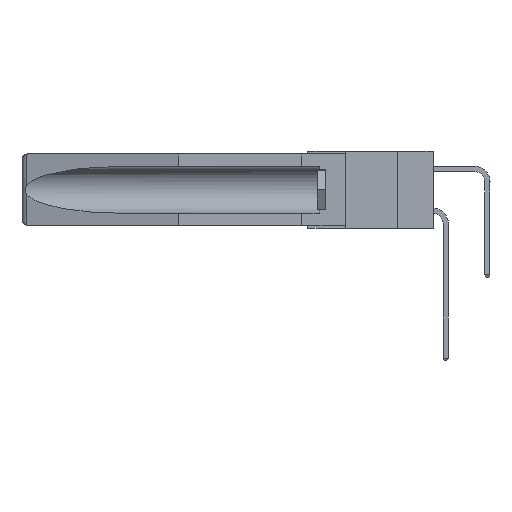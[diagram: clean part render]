
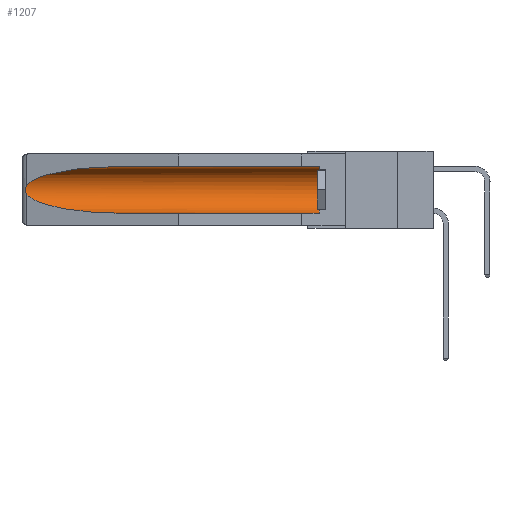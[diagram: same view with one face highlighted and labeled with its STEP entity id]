
A CAD part, left-side view. The second image highlights one B-rep face of the part: STEP entity #1207.
In plain terms, the highlighted cylindrical face has radius 2.857 mm (diameter 5.715 mm), a partial arc.
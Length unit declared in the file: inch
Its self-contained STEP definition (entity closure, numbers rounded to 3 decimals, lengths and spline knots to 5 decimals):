
#34 = CARTESIAN_POINT ( 'NONE',  ( 0.26655, 1.53094, -0.18657 ) ) ;
#533 = CARTESIAN_POINT ( 'NONE',  ( 0.155, 0.126, -0.059 ) ) ;
#949 = VERTEX_POINT ( 'NONE', #533 ) ;
#1207 = ADVANCED_FACE ( 'NONE', ( #13587 ), #18094, .F. ) ;
#1310 = CARTESIAN_POINT ( 'NONE',  ( 0.155, 0.126, -0.284 ) ) ;
#1577 = CARTESIAN_POINT ( 'NONE',  ( 0.26597, 1.5296, -0.19026 ) ) ;
#2385 = CARTESIAN_POINT ( 'NONE',  ( 0.155, 1.07973, -0.059 ) ) ;
#2899 = CARTESIAN_POINT ( 'NONE',  ( 0.2675, 1.53308, -0.16763 ) ) ;
#3165 = CARTESIAN_POINT ( 'NONE',  ( 0.26597, 1.52961, -0.15275 ) ) ;
#3187 =( BOUNDED_CURVE ( )  B_SPLINE_CURVE ( 3, ( #5237, #18400, #6705, #9602 ),
 .UNSPECIFIED., .F., .F. ) 
 B_SPLINE_CURVE_WITH_KNOTS ( ( 4, 4 ),
 ( 0.1948, 1.5708 ),
 .UNSPECIFIED. ) 
 CURVE ( )  GEOMETRIC_REPRESENTATION_ITEM ( )  RATIONAL_B_SPLINE_CURVE ( ( 1., 0.848, 0.848, 1. ) ) 
 REPRESENTATION_ITEM ( '' )  );
#3594 = ORIENTED_EDGE ( 'NONE', *, *, #14632, .T. ) ;
#4038 = CARTESIAN_POINT ( 'NONE',  ( 0.155, 1.07973, -0.059 ) ) ;
#4107 = DIRECTION ( 'NONE',  ( 0., 0., 1. ) ) ;
#4496 = CARTESIAN_POINT ( 'NONE',  ( 0.26537, 1.52718, -0.19328 ) ) ;
#5037 = CIRCLE ( 'NONE', #17253, 0.1125 ) ;
#5213 = ORIENTED_EDGE ( 'NONE', *, *, #16101, .T. ) ;
#5237 = CARTESIAN_POINT ( 'NONE',  ( 0.26537, 1.52718, -0.19328 ) ) ;
#5272 = CARTESIAN_POINT ( 'NONE',  ( 0.21114, 1.30732, -0.059 ) ) ;
#6705 = CARTESIAN_POINT ( 'NONE',  ( 0.21114, 1.30732, -0.284 ) ) ;
#7169 = VERTEX_POINT ( 'NONE', #14437 ) ;
#7429 = CARTESIAN_POINT ( 'NONE',  ( 0.155, -0.30754, -0.1715 ) ) ;
#7933 = CARTESIAN_POINT ( 'NONE',  ( 0.155, -0.30754, -0.284 ) ) ;
#8153 = CARTESIAN_POINT ( 'NONE',  ( 0.26537, 1.52718, -0.14972 ) ) ;
#8273 = CARTESIAN_POINT ( 'NONE',  ( 0.25451, 1.48313, -0.09465 ) ) ;
#8416 = EDGE_CURVE ( 'NONE', #9540, #18323, #3187, .T. ) ;
#8441 = ORIENTED_EDGE ( 'NONE', *, *, #12643, .T. ) ;
#8804 = DIRECTION ( 'NONE',  ( 0., 0., 1. ) ) ;
#9417 = VECTOR ( 'NONE', #18021, 39.37008 ) ;
#9540 = VERTEX_POINT ( 'NONE', #13170 ) ;
#9602 = CARTESIAN_POINT ( 'NONE',  ( 0.155, 1.07973, -0.284 ) ) ;
#9893 = DIRECTION ( 'NONE',  ( 0., -1., 0. ) ) ;
#10292 = CARTESIAN_POINT ( 'NONE',  ( 0.2673, 1.53269, -0.17917 ) ) ;
#10421 = CARTESIAN_POINT ( 'NONE',  ( 0.2675, 1.53308, -0.17534 ) ) ;
#11220 = ORIENTED_EDGE ( 'NONE', *, *, #12162, .F. ) ;
#11385 = B_SPLINE_CURVE_WITH_KNOTS ( 'NONE', 3,
 ( #17722, #3165, #17658, #13363, #2899, #10421, #10292, #34, #1577, #4496 ),
 .UNSPECIFIED., .F., .F.,
 ( 4, 2, 2, 2, 4 ),
 ( 0., 0.00029, 0.00058, 0.00087, 0.00117 ),
 .UNSPECIFIED. ) ;
#11499 = CARTESIAN_POINT ( 'NONE',  ( 0.155, 0.126, -0.1715 ) ) ;
#11554 = EDGE_CURVE ( 'NONE', #949, #14743, #14263, .T. ) ;
#12162 = EDGE_CURVE ( 'NONE', #16136, #18323, #17405, .T. ) ;
#12643 = EDGE_CURVE ( 'NONE', #7169, #9540, #11385, .T. ) ;
#13170 = CARTESIAN_POINT ( 'NONE',  ( 0.26537, 1.52718, -0.19328 ) ) ;
#13363 = CARTESIAN_POINT ( 'NONE',  ( 0.2673, 1.5327, -0.16383 ) ) ;
#13423 = EDGE_LOOP ( 'NONE', ( #3594, #8441, #16277, #11220, #5213, #15487 ) ) ;
#13587 = FACE_OUTER_BOUND ( 'NONE', #13423, .T. ) ;
#14263 = LINE ( 'NONE', #18414, #15396 ) ;
#14437 = CARTESIAN_POINT ( 'NONE',  ( 0.26537, 1.52718, -0.14972 ) ) ;
#14626 = CARTESIAN_POINT ( 'NONE',  ( 0.155, 1.07973, -0.284 ) ) ;
#14632 = EDGE_CURVE ( 'NONE', #14743, #7169, #17813, .T. ) ;
#14743 = VERTEX_POINT ( 'NONE', #2385 ) ;
#14782 = DIRECTION ( 'NONE',  ( 0., 1., 0. ) ) ;
#15396 = VECTOR ( 'NONE', #18229, 39.37008 ) ;
#15487 = ORIENTED_EDGE ( 'NONE', *, *, #11554, .T. ) ;
#16101 = EDGE_CURVE ( 'NONE', #16136, #949, #5037, .T. ) ;
#16136 = VERTEX_POINT ( 'NONE', #1310 ) ;
#16277 = ORIENTED_EDGE ( 'NONE', *, *, #8416, .T. ) ;
#16861 = AXIS2_PLACEMENT_3D ( 'NONE', #7429, #14782, #8804 ) ;
#17253 = AXIS2_PLACEMENT_3D ( 'NONE', #11499, #9893, #4107 ) ;
#17405 = LINE ( 'NONE', #7933, #9417 ) ;
#17658 = CARTESIAN_POINT ( 'NONE',  ( 0.26654, 1.53092, -0.15636 ) ) ;
#17722 = CARTESIAN_POINT ( 'NONE',  ( 0.26537, 1.52718, -0.14972 ) ) ;
#17813 =( BOUNDED_CURVE ( )  B_SPLINE_CURVE ( 3, ( #4038, #5272, #8273, #8153 ),
 .UNSPECIFIED., .F., .F. ) 
 B_SPLINE_CURVE_WITH_KNOTS ( ( 4, 4 ),
 ( 4.71239, 6.08839 ),
 .UNSPECIFIED. ) 
 CURVE ( )  GEOMETRIC_REPRESENTATION_ITEM ( )  RATIONAL_B_SPLINE_CURVE ( ( 1., 0.848, 0.848, 1. ) ) 
 REPRESENTATION_ITEM ( '' )  );
#18021 = DIRECTION ( 'NONE',  ( 0., 1., 0. ) ) ;
#18094 = CYLINDRICAL_SURFACE ( 'NONE', #16861, 0.1125 ) ;
#18229 = DIRECTION ( 'NONE',  ( 0., 1., 0. ) ) ;
#18323 = VERTEX_POINT ( 'NONE', #14626 ) ;
#18400 = CARTESIAN_POINT ( 'NONE',  ( 0.25451, 1.48313, -0.24835 ) ) ;
#18414 = CARTESIAN_POINT ( 'NONE',  ( 0.155, -0.30754, -0.059 ) ) ;
